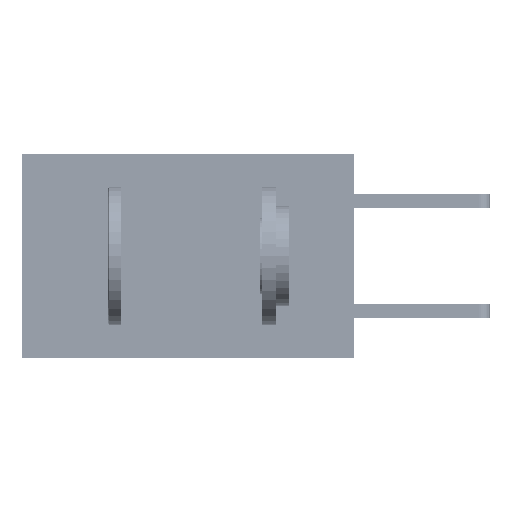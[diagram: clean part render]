
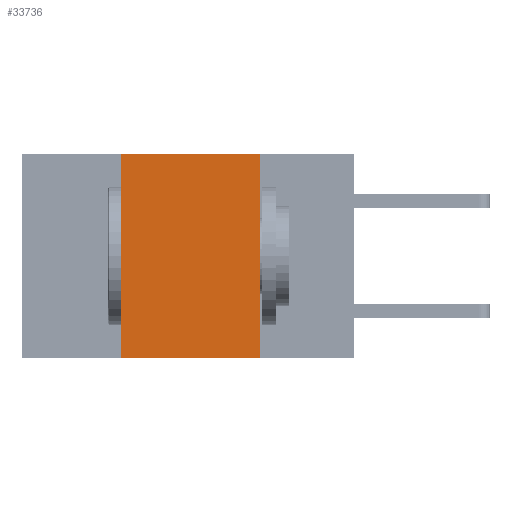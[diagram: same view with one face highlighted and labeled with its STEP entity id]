
A CAD part, left-side view. The second image highlights one B-rep face of the part: STEP entity #33736.
In plain terms, the highlighted planar face has unit normal (-1, 0, 0).
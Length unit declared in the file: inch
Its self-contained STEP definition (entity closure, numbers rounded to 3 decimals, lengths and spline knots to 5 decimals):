
#2480 = ORIENTED_EDGE ( 'NONE', *, *, #5294, .T. ) ;
#2604 = DIRECTION ( 'NONE',  ( 0., -1., 0. ) ) ;
#3048 = DIRECTION ( 'NONE',  ( 0., 0., -1. ) ) ;
#3531 = LINE ( 'NONE', #29943, #40123 ) ;
#5159 = DIRECTION ( 'NONE',  ( 1., 0., 0. ) ) ;
#5294 = EDGE_CURVE ( 'NONE', #23550, #26106, #33594, .T. ) ;
#9270 = DIRECTION ( 'NONE',  ( 0., 0., -1. ) ) ;
#11128 = EDGE_CURVE ( 'NONE', #23550, #38050, #12687, .T. ) ;
#11636 = VECTOR ( 'NONE', #20872, 39.37008 ) ;
#12687 = LINE ( 'NONE', #16769, #11636 ) ;
#13862 = FACE_OUTER_BOUND ( 'NONE', #50048, .T. ) ;
#16769 = CARTESIAN_POINT ( 'NONE',  ( 0., 0.42, 0. ) ) ;
#17722 = PLANE ( 'NONE',  #43915 ) ;
#18720 = ORIENTED_EDGE ( 'NONE', *, *, #38183, .F. ) ;
#19201 = ORIENTED_EDGE ( 'NONE', *, *, #11128, .F. ) ;
#20494 = VECTOR ( 'NONE', #2604, 39.37008 ) ;
#20872 = DIRECTION ( 'NONE',  ( 0., 0., 1. ) ) ;
#21284 = CARTESIAN_POINT ( 'NONE',  ( 0., 0.6, 0. ) ) ;
#23397 = EDGE_CURVE ( 'NONE', #35762, #26106, #3531, .T. ) ;
#23550 = VERTEX_POINT ( 'NONE', #35283 ) ;
#25801 = DIRECTION ( 'NONE',  ( 0., -1., 0. ) ) ;
#26106 = VERTEX_POINT ( 'NONE', #27591 ) ;
#27591 = CARTESIAN_POINT ( 'NONE',  ( 0., 0.17, -0.37 ) ) ;
#28617 = CARTESIAN_POINT ( 'NONE',  ( 0., 0.42, 0. ) ) ;
#29943 = CARTESIAN_POINT ( 'NONE',  ( 0., 0.17, 0. ) ) ;
#32250 = VECTOR ( 'NONE', #25801, 39.37008 ) ;
#33594 = LINE ( 'NONE', #38218, #20494 ) ;
#33733 = CARTESIAN_POINT ( 'NONE',  ( 0., 0.6, 0. ) ) ;
#33736 = ADVANCED_FACE ( 'NONE', ( #13862 ), #17722, .F. ) ;
#35283 = CARTESIAN_POINT ( 'NONE',  ( 0., 0.42, -0.37 ) ) ;
#35762 = VERTEX_POINT ( 'NONE', #50142 ) ;
#38050 = VERTEX_POINT ( 'NONE', #28617 ) ;
#38183 = EDGE_CURVE ( 'NONE', #38050, #35762, #49112, .T. ) ;
#38218 = CARTESIAN_POINT ( 'NONE',  ( 0., 0.6, -0.37 ) ) ;
#40123 = VECTOR ( 'NONE', #3048, 39.37008 ) ;
#43915 = AXIS2_PLACEMENT_3D ( 'NONE', #21284, #5159, #9270 ) ;
#46278 = ORIENTED_EDGE ( 'NONE', *, *, #23397, .F. ) ;
#49112 = LINE ( 'NONE', #33733, #32250 ) ;
#50048 = EDGE_LOOP ( 'NONE', ( #46278, #18720, #19201, #2480 ) ) ;
#50142 = CARTESIAN_POINT ( 'NONE',  ( 0., 0.17, 0. ) ) ;
